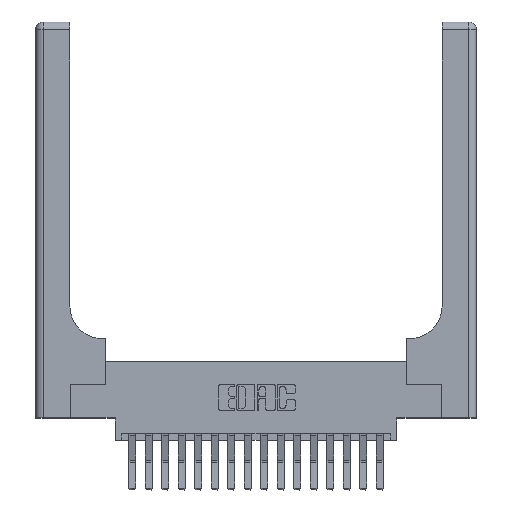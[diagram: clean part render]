
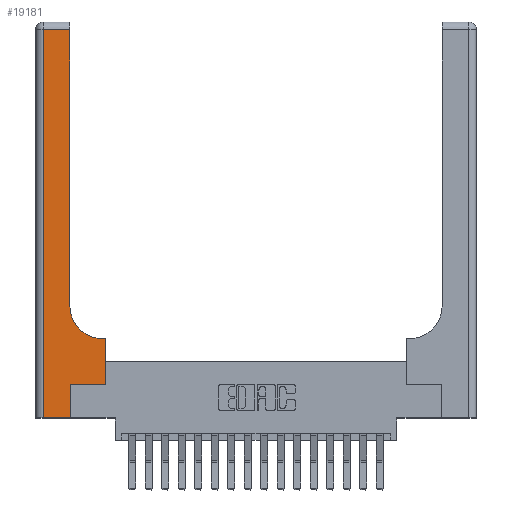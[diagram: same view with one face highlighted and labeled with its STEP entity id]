
A CAD part, top view. The second image highlights one B-rep face of the part: STEP entity #19181.
In plain terms, the highlighted planar face has unit normal (0, 0, 1).
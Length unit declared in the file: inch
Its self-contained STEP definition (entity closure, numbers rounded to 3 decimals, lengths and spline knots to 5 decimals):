
#60 = CARTESIAN_POINT ( 'NONE',  ( 0.26, 0.6, 0.37 ) ) ;
#141 = DIRECTION ( 'NONE',  ( 0., 0., -1. ) ) ;
#288 = VECTOR ( 'NONE', #11773, 39.37008 ) ;
#303 = VERTEX_POINT ( 'NONE', #5223 ) ;
#463 = VECTOR ( 'NONE', #14041, 39.37008 ) ;
#762 = LINE ( 'NONE', #5653, #288 ) ;
#1553 = DIRECTION ( 'NONE',  ( -1., 0., 0. ) ) ;
#2535 = VECTOR ( 'NONE', #5352, 39.37008 ) ;
#2730 = VERTEX_POINT ( 'NONE', #19301 ) ;
#2880 = EDGE_CURVE ( 'NONE', #2730, #9452, #10711, .T. ) ;
#3028 = FACE_OUTER_BOUND ( 'NONE', #11151, .T. ) ;
#3466 = EDGE_CURVE ( 'NONE', #3560, #303, #6253, .T. ) ;
#3480 = ORIENTED_EDGE ( 'NONE', *, *, #3466, .T. ) ;
#3560 = VERTEX_POINT ( 'NONE', #17849 ) ;
#3623 = DIRECTION ( 'NONE',  ( -1., 0., 0. ) ) ;
#4560 = EDGE_CURVE ( 'NONE', #9452, #14811, #7850, .T. ) ;
#4870 = CARTESIAN_POINT ( 'NONE',  ( 0.06, 2.94, 0.37 ) ) ;
#5223 = CARTESIAN_POINT ( 'NONE',  ( 0.528, 0.25, 0.37 ) ) ;
#5351 = CARTESIAN_POINT ( 'NONE',  ( 0.06, 0., 0.37 ) ) ;
#5352 = DIRECTION ( 'NONE',  ( 1., 0., 0. ) ) ;
#5488 = ORIENTED_EDGE ( 'NONE', *, *, #18854, .T. ) ;
#5653 = CARTESIAN_POINT ( 'NONE',  ( 0.26, 3., 0.37 ) ) ;
#5656 = CARTESIAN_POINT ( 'NONE',  ( 0.26, 0.85, 0.37 ) ) ;
#6149 = CARTESIAN_POINT ( 'NONE',  ( 0.265, 0., 0.37 ) ) ;
#6245 = ORIENTED_EDGE ( 'NONE', *, *, #12247, .T. ) ;
#6253 = LINE ( 'NONE', #6644, #463 ) ;
#6348 = DIRECTION ( 'NONE',  ( 0., -1., 0. ) ) ;
#6600 = VERTEX_POINT ( 'NONE', #7392 ) ;
#6644 = CARTESIAN_POINT ( 'NONE',  ( 0.265, 0.25, 0.37 ) ) ;
#6773 = VECTOR ( 'NONE', #6348, 39.37008 ) ;
#7392 = CARTESIAN_POINT ( 'NONE',  ( 0.26, 2.94, 0.37 ) ) ;
#7464 = DIRECTION ( 'NONE',  ( 1., 0., 0. ) ) ;
#7756 = PLANE ( 'NONE',  #11267 ) ;
#7850 = CIRCLE ( 'NONE', #18092, 0.25 ) ;
#8086 = VERTEX_POINT ( 'NONE', #4870 ) ;
#8889 = CARTESIAN_POINT ( 'NONE',  ( 0.51, 0.85, 0.37 ) ) ;
#9452 = VERTEX_POINT ( 'NONE', #18096 ) ;
#9630 = LINE ( 'NONE', #6149, #13780 ) ;
#9764 = CARTESIAN_POINT ( 'NONE',  ( 0.06, 3., 0.37 ) ) ;
#9808 = VERTEX_POINT ( 'NONE', #5351 ) ;
#10210 = ORIENTED_EDGE ( 'NONE', *, *, #19189, .T. ) ;
#10652 = EDGE_CURVE ( 'NONE', #14811, #6600, #762, .T. ) ;
#10711 = LINE ( 'NONE', #60, #11489 ) ;
#11151 = EDGE_LOOP ( 'NONE', ( #14609, #6245, #14981, #5488, #10210, #3480, #18891, #19512, #13880 ) ) ;
#11177 = LINE ( 'NONE', #9764, #6773 ) ;
#11267 = AXIS2_PLACEMENT_3D ( 'NONE', #18478, #18836, #18276 ) ;
#11489 = VECTOR ( 'NONE', #1553, 39.37008 ) ;
#11773 = DIRECTION ( 'NONE',  ( 0., 1., 0. ) ) ;
#12247 = EDGE_CURVE ( 'NONE', #6600, #8086, #12751, .T. ) ;
#12364 = LINE ( 'NONE', #18178, #14106 ) ;
#12751 = LINE ( 'NONE', #18870, #17599 ) ;
#13559 = CARTESIAN_POINT ( 'NONE',  ( 0.265, 0., 0.37 ) ) ;
#13780 = VECTOR ( 'NONE', #15810, 39.37008 ) ;
#13880 = ORIENTED_EDGE ( 'NONE', *, *, #4560, .T. ) ;
#14041 = DIRECTION ( 'NONE',  ( 1., 0., 0. ) ) ;
#14106 = VECTOR ( 'NONE', #18491, 39.37008 ) ;
#14358 = LINE ( 'NONE', #17461, #2535 ) ;
#14609 = ORIENTED_EDGE ( 'NONE', *, *, #10652, .T. ) ;
#14811 = VERTEX_POINT ( 'NONE', #5656 ) ;
#14981 = ORIENTED_EDGE ( 'NONE', *, *, #15169, .T. ) ;
#15025 = EDGE_CURVE ( 'NONE', #303, #2730, #12364, .T. ) ;
#15169 = EDGE_CURVE ( 'NONE', #8086, #9808, #11177, .T. ) ;
#15810 = DIRECTION ( 'NONE',  ( 0., 1., 0. ) ) ;
#16250 = VERTEX_POINT ( 'NONE', #13559 ) ;
#17461 = CARTESIAN_POINT ( 'NONE',  ( 0., 0., 0.37 ) ) ;
#17599 = VECTOR ( 'NONE', #3623, 39.37008 ) ;
#17849 = CARTESIAN_POINT ( 'NONE',  ( 0.265, 0.25, 0.37 ) ) ;
#18092 = AXIS2_PLACEMENT_3D ( 'NONE', #8889, #141, #7464 ) ;
#18096 = CARTESIAN_POINT ( 'NONE',  ( 0.51, 0.6, 0.37 ) ) ;
#18178 = CARTESIAN_POINT ( 'NONE',  ( 0.528, 0.25, 0.37 ) ) ;
#18276 = DIRECTION ( 'NONE',  ( -1., 0., 0. ) ) ;
#18478 = CARTESIAN_POINT ( 'NONE',  ( 0., 3., 0.37 ) ) ;
#18491 = DIRECTION ( 'NONE',  ( 0., 1., 0. ) ) ;
#18836 = DIRECTION ( 'NONE',  ( 0., 0., -1. ) ) ;
#18854 = EDGE_CURVE ( 'NONE', #9808, #16250, #14358, .T. ) ;
#18870 = CARTESIAN_POINT ( 'NONE',  ( 0., 2.94, 0.37 ) ) ;
#18891 = ORIENTED_EDGE ( 'NONE', *, *, #15025, .T. ) ;
#19181 = ADVANCED_FACE ( 'NONE', ( #3028 ), #7756, .F. ) ;
#19189 = EDGE_CURVE ( 'NONE', #16250, #3560, #9630, .T. ) ;
#19301 = CARTESIAN_POINT ( 'NONE',  ( 0.528, 0.6, 0.37 ) ) ;
#19512 = ORIENTED_EDGE ( 'NONE', *, *, #2880, .T. ) ;
